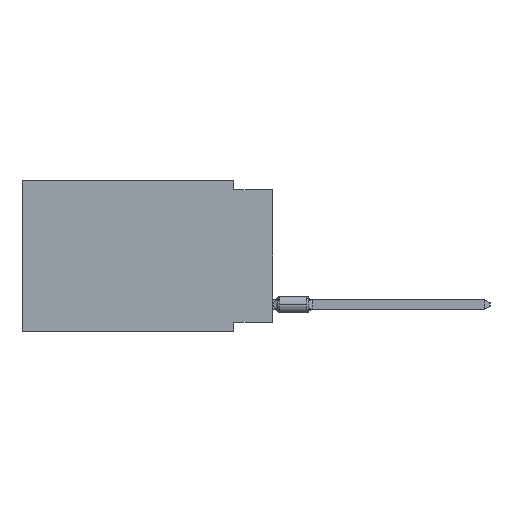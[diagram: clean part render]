
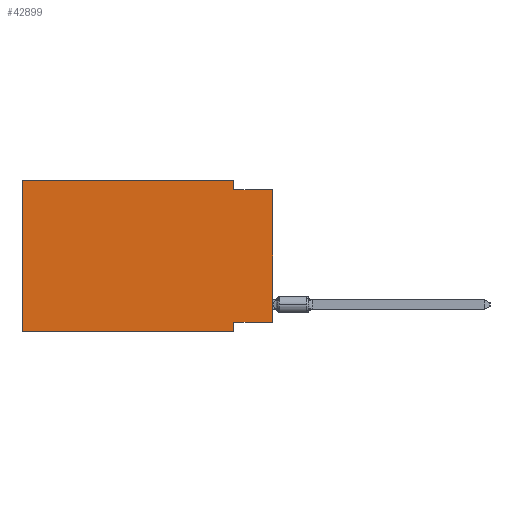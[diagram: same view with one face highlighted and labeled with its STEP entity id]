
A CAD part, left-side view. The second image highlights one B-rep face of the part: STEP entity #42899.
In plain terms, the highlighted planar face has unit normal (-1, 0, 0).
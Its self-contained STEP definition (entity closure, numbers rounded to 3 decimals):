
#569 = LINE ( 'NONE', #46627, #40225 ) ;
#3148 = PLANE ( 'NONE',  #40077 ) ;
#3269 = LINE ( 'NONE', #14360, #38071 ) ;
#4260 = LINE ( 'NONE', #42525, #26537 ) ;
#5914 = CARTESIAN_POINT ( 'NONE',  ( 0., 0., -0.635 ) ) ;
#7291 = DIRECTION ( 'NONE',  ( 0., 0., 1. ) ) ;
#7963 = EDGE_CURVE ( 'NONE', #45836, #26290, #569, .T. ) ;
#8515 = DIRECTION ( 'NONE',  ( 0., -1., 0. ) ) ;
#9169 = DIRECTION ( 'NONE',  ( 0., -1., 0. ) ) ;
#9806 = CARTESIAN_POINT ( 'NONE',  ( 0., 2.54, -9.906 ) ) ;
#10025 = LINE ( 'NONE', #17600, #48370 ) ;
#10570 = VECTOR ( 'NONE', #7291, 1000. ) ;
#10697 = CARTESIAN_POINT ( 'NONE',  ( 0., 16.383, 0. ) ) ;
#10801 = ORIENTED_EDGE ( 'NONE', *, *, #13431, .F. ) ;
#11084 = EDGE_CURVE ( 'NONE', #32981, #30809, #38009, .T. ) ;
#12003 = VECTOR ( 'NONE', #43432, 1000. ) ;
#12019 = ORIENTED_EDGE ( 'NONE', *, *, #23735, .F. ) ;
#12947 = VERTEX_POINT ( 'NONE', #32634 ) ;
#13431 = EDGE_CURVE ( 'NONE', #30285, #45836, #20518, .T. ) ;
#14050 = CARTESIAN_POINT ( 'NONE',  ( 0., 16.383, 0. ) ) ;
#14360 = CARTESIAN_POINT ( 'NONE',  ( 0., 2.54, -9.906 ) ) ;
#14461 = VECTOR ( 'NONE', #21302, 1000. ) ;
#17522 = LINE ( 'NONE', #5914, #14461 ) ;
#17600 = CARTESIAN_POINT ( 'NONE',  ( 0., 16.383, 0. ) ) ;
#17768 = EDGE_LOOP ( 'NONE', ( #27083, #20108, #25926, #10801, #48966, #34159, #49301, #12019 ) ) ;
#18911 = CARTESIAN_POINT ( 'NONE',  ( 0., 2.54, 0. ) ) ;
#20108 = ORIENTED_EDGE ( 'NONE', *, *, #44051, .F. ) ;
#20210 = CARTESIAN_POINT ( 'NONE',  ( 0., 0., -0.635 ) ) ;
#20222 = DIRECTION ( 'NONE',  ( 0., 0., -1. ) ) ;
#20518 = LINE ( 'NONE', #43661, #49448 ) ;
#21302 = DIRECTION ( 'NONE',  ( 0., -1., 0. ) ) ;
#22513 = CARTESIAN_POINT ( 'NONE',  ( 0., 2.54, -0.635 ) ) ;
#23589 = CARTESIAN_POINT ( 'NONE',  ( 0., 0., -9.271 ) ) ;
#23735 = EDGE_CURVE ( 'NONE', #32981, #30965, #24314, .T. ) ;
#24314 = LINE ( 'NONE', #23589, #12003 ) ;
#24716 = CARTESIAN_POINT ( 'NONE',  ( 0., 2.54, -9.271 ) ) ;
#25926 = ORIENTED_EDGE ( 'NONE', *, *, #7963, .F. ) ;
#26290 = VERTEX_POINT ( 'NONE', #22513 ) ;
#26537 = VECTOR ( 'NONE', #8515, 1000. ) ;
#27083 = ORIENTED_EDGE ( 'NONE', *, *, #11084, .T. ) ;
#28415 = DIRECTION ( 'NONE',  ( 0., 0., 1. ) ) ;
#29825 = DIRECTION ( 'NONE',  ( 0., 0., -1. ) ) ;
#30285 = VERTEX_POINT ( 'NONE', #14050 ) ;
#30599 = CARTESIAN_POINT ( 'NONE',  ( 0., 0., -9.271 ) ) ;
#30809 = VERTEX_POINT ( 'NONE', #20210 ) ;
#30965 = VERTEX_POINT ( 'NONE', #24716 ) ;
#31318 = EDGE_CURVE ( 'NONE', #12947, #30285, #10025, .T. ) ;
#32634 = CARTESIAN_POINT ( 'NONE',  ( 0., 16.383, -9.906 ) ) ;
#32981 = VERTEX_POINT ( 'NONE', #30599 ) ;
#33501 = CARTESIAN_POINT ( 'NONE',  ( 0., 0., 0. ) ) ;
#33611 = EDGE_CURVE ( 'NONE', #30965, #35180, #3269, .T. ) ;
#33741 = DIRECTION ( 'NONE',  ( 0., 0., -1. ) ) ;
#34159 = ORIENTED_EDGE ( 'NONE', *, *, #39964, .T. ) ;
#35180 = VERTEX_POINT ( 'NONE', #9806 ) ;
#38009 = LINE ( 'NONE', #33501, #10570 ) ;
#38071 = VECTOR ( 'NONE', #33741, 1000. ) ;
#39964 = EDGE_CURVE ( 'NONE', #12947, #35180, #4260, .T. ) ;
#40077 = AXIS2_PLACEMENT_3D ( 'NONE', #10697, #45173, #29825 ) ;
#40225 = VECTOR ( 'NONE', #20222, 1000. ) ;
#42525 = CARTESIAN_POINT ( 'NONE',  ( 0., 16.383, -9.906 ) ) ;
#42899 = ADVANCED_FACE ( 'NONE', ( #46170 ), #3148, .F. ) ;
#43432 = DIRECTION ( 'NONE',  ( 0., 1., 0. ) ) ;
#43661 = CARTESIAN_POINT ( 'NONE',  ( 0., 16.383, 0. ) ) ;
#44051 = EDGE_CURVE ( 'NONE', #26290, #30809, #17522, .T. ) ;
#45173 = DIRECTION ( 'NONE',  ( 1., 0., 0. ) ) ;
#45836 = VERTEX_POINT ( 'NONE', #18911 ) ;
#46170 = FACE_OUTER_BOUND ( 'NONE', #17768, .T. ) ;
#46627 = CARTESIAN_POINT ( 'NONE',  ( 0., 2.54, 0. ) ) ;
#48370 = VECTOR ( 'NONE', #28415, 1000. ) ;
#48966 = ORIENTED_EDGE ( 'NONE', *, *, #31318, .F. ) ;
#49301 = ORIENTED_EDGE ( 'NONE', *, *, #33611, .F. ) ;
#49448 = VECTOR ( 'NONE', #9169, 1000. ) ;
